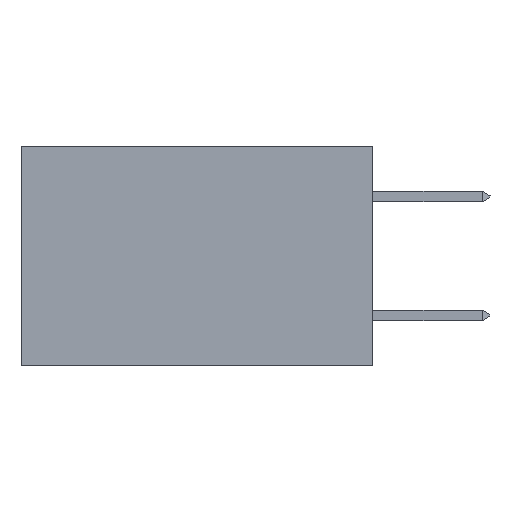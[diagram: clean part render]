
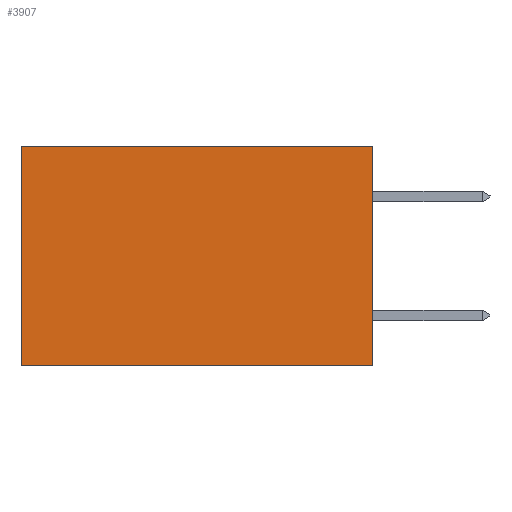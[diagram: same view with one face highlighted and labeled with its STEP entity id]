
A CAD part, left-side view. The second image highlights one B-rep face of the part: STEP entity #3907.
In plain terms, the highlighted planar face has unit normal (-1, 0, 0).
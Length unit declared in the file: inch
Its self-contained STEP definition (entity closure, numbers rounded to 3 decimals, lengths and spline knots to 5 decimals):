
#58 = CARTESIAN_POINT ( 'NONE',  ( 0.277, 0., -0.37 ) ) ;
#104 = DIRECTION ( 'NONE',  ( 0., 0., -1. ) ) ;
#469 = ORIENTED_EDGE ( 'NONE', *, *, #11088, .F. ) ;
#1381 = AXIS2_PLACEMENT_3D ( 'NONE', #4306, #4061, #11211 ) ;
#1477 = DIRECTION ( 'NONE',  ( 0., 1., 0. ) ) ;
#1478 = CARTESIAN_POINT ( 'NONE',  ( 0.277, 0., 0. ) ) ;
#2006 = ORIENTED_EDGE ( 'NONE', *, *, #5454, .F. ) ;
#2810 = VERTEX_POINT ( 'NONE', #3407 ) ;
#3230 = CARTESIAN_POINT ( 'NONE',  ( 0.277, 0., -0.37 ) ) ;
#3407 = CARTESIAN_POINT ( 'NONE',  ( 0.277, 0.59, 0. ) ) ;
#3603 = ORIENTED_EDGE ( 'NONE', *, *, #3695, .T. ) ;
#3695 = EDGE_CURVE ( 'NONE', #2810, #6144, #9484, .T. ) ;
#3903 = VECTOR ( 'NONE', #1477, 39.37008 ) ;
#3907 = ADVANCED_FACE ( 'NONE', ( #7275 ), #8448, .F. ) ;
#4061 = DIRECTION ( 'NONE',  ( 1., 0., 0. ) ) ;
#4306 = CARTESIAN_POINT ( 'NONE',  ( 0.277, 0., -0.37 ) ) ;
#4679 = CARTESIAN_POINT ( 'NONE',  ( 0.277, 0., 0. ) ) ;
#4700 = VERTEX_POINT ( 'NONE', #1478 ) ;
#5248 = DIRECTION ( 'NONE',  ( 0., 1., 0. ) ) ;
#5454 = EDGE_CURVE ( 'NONE', #9308, #6144, #5576, .T. ) ;
#5553 = EDGE_CURVE ( 'NONE', #4700, #2810, #7349, .T. ) ;
#5576 = LINE ( 'NONE', #3230, #10683 ) ;
#6124 = LINE ( 'NONE', #58, #7084 ) ;
#6144 = VERTEX_POINT ( 'NONE', #7608 ) ;
#6788 = VECTOR ( 'NONE', #8162, 39.37008 ) ;
#7084 = VECTOR ( 'NONE', #104, 39.37008 ) ;
#7275 = FACE_OUTER_BOUND ( 'NONE', #8989, .T. ) ;
#7349 = LINE ( 'NONE', #4679, #3903 ) ;
#7608 = CARTESIAN_POINT ( 'NONE',  ( 0.277, 0.59, -0.37 ) ) ;
#8162 = DIRECTION ( 'NONE',  ( 0., 0., -1. ) ) ;
#8339 = ORIENTED_EDGE ( 'NONE', *, *, #5553, .T. ) ;
#8448 = PLANE ( 'NONE',  #1381 ) ;
#8989 = EDGE_LOOP ( 'NONE', ( #3603, #2006, #469, #8339 ) ) ;
#9033 = CARTESIAN_POINT ( 'NONE',  ( 0.277, 0., -0.37 ) ) ;
#9308 = VERTEX_POINT ( 'NONE', #9033 ) ;
#9484 = LINE ( 'NONE', #12497, #6788 ) ;
#10683 = VECTOR ( 'NONE', #5248, 39.37008 ) ;
#11088 = EDGE_CURVE ( 'NONE', #4700, #9308, #6124, .T. ) ;
#11211 = DIRECTION ( 'NONE',  ( 0., 0., -1. ) ) ;
#12497 = CARTESIAN_POINT ( 'NONE',  ( 0.277, 0.59, -0.37 ) ) ;
